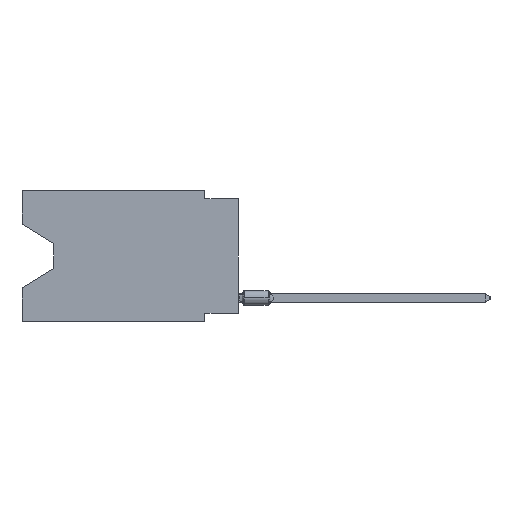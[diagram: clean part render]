
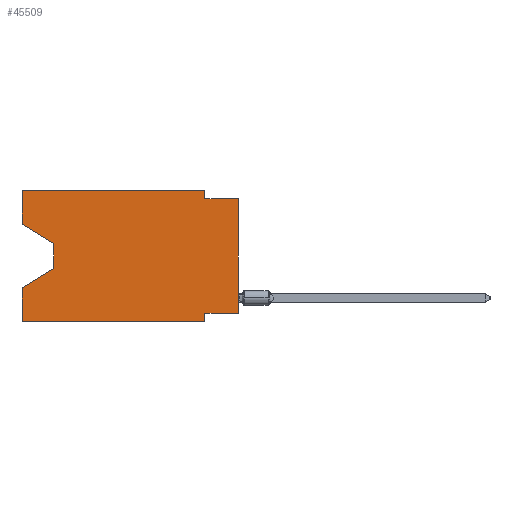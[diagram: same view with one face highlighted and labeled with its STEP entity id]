
A CAD part, left-side view. The second image highlights one B-rep face of the part: STEP entity #45509.
In plain terms, the highlighted planar face has unit normal (-1, 0, 0).
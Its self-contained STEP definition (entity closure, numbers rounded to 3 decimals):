
#133 = DIRECTION ( 'NONE',  ( 0., 0., -1. ) ) ;
#1844 = CARTESIAN_POINT ( 'NONE',  ( 0., 16.383, -2.546 ) ) ;
#2037 = ORIENTED_EDGE ( 'NONE', *, *, #19063, .T. ) ;
#2393 = CARTESIAN_POINT ( 'NONE',  ( 0., 0., -9.271 ) ) ;
#4251 = ORIENTED_EDGE ( 'NONE', *, *, #30617, .T. ) ;
#4697 = LINE ( 'NONE', #22172, #10840 ) ;
#5427 = VECTOR ( 'NONE', #28381, 1000. ) ;
#6247 = DIRECTION ( 'NONE',  ( 0., -1., 0. ) ) ;
#6946 = DIRECTION ( 'NONE',  ( 0., 1., 0. ) ) ;
#7631 = LINE ( 'NONE', #42583, #11906 ) ;
#7999 = CARTESIAN_POINT ( 'NONE',  ( 0., 16.383, 0. ) ) ;
#8309 = CARTESIAN_POINT ( 'NONE',  ( 0., 2.54, -9.906 ) ) ;
#9301 = LINE ( 'NONE', #1844, #46509 ) ;
#9688 = CARTESIAN_POINT ( 'NONE',  ( 0., 16.383, -2.546 ) ) ;
#10560 = LINE ( 'NONE', #45496, #26083 ) ;
#10840 = VECTOR ( 'NONE', #40492, 1000. ) ;
#11053 = ORIENTED_EDGE ( 'NONE', *, *, #41246, .F. ) ;
#11726 = DIRECTION ( 'NONE',  ( 0., 0., -1. ) ) ;
#11906 = VECTOR ( 'NONE', #54344, 1000. ) ;
#12915 = EDGE_CURVE ( 'NONE', #19166, #28089, #10560, .T. ) ;
#14670 = VECTOR ( 'NONE', #133, 1000. ) ;
#16348 = PLANE ( 'NONE',  #28451 ) ;
#17583 = VECTOR ( 'NONE', #33090, 1000. ) ;
#17687 = EDGE_CURVE ( 'NONE', #28089, #47008, #52532, .T. ) ;
#18298 = VERTEX_POINT ( 'NONE', #21334 ) ;
#19063 = EDGE_CURVE ( 'NONE', #41178, #54456, #50975, .T. ) ;
#19128 = CARTESIAN_POINT ( 'NONE',  ( 0., 2.54, 0. ) ) ;
#19166 = VERTEX_POINT ( 'NONE', #7999 ) ;
#19628 = LINE ( 'NONE', #37091, #17583 ) ;
#19798 = EDGE_CURVE ( 'NONE', #53933, #18298, #41623, .T. ) ;
#20090 = VECTOR ( 'NONE', #25200, 1000. ) ;
#20174 = VECTOR ( 'NONE', #6946, 1000. ) ;
#20194 = CARTESIAN_POINT ( 'NONE',  ( 0., 2.54, -0.635 ) ) ;
#20821 = CARTESIAN_POINT ( 'NONE',  ( 0., 16.383, -9.906 ) ) ;
#21334 = CARTESIAN_POINT ( 'NONE',  ( 0., 2.54, -9.271 ) ) ;
#21633 = VERTEX_POINT ( 'NONE', #9688 ) ;
#21896 = CARTESIAN_POINT ( 'NONE',  ( 0., 2.54, 0. ) ) ;
#22172 = CARTESIAN_POINT ( 'NONE',  ( 0., 0., -0.635 ) ) ;
#22261 = ORIENTED_EDGE ( 'NONE', *, *, #12915, .F. ) ;
#22433 = LINE ( 'NONE', #27019, #33358 ) ;
#22599 = CARTESIAN_POINT ( 'NONE',  ( 0., 16.383, -7.36 ) ) ;
#23037 = ORIENTED_EDGE ( 'NONE', *, *, #19798, .F. ) ;
#23476 = VERTEX_POINT ( 'NONE', #24173 ) ;
#23794 = LINE ( 'NONE', #28670, #5427 ) ;
#24173 = CARTESIAN_POINT ( 'NONE',  ( 0., 0., -0.635 ) ) ;
#24440 = EDGE_CURVE ( 'NONE', #53933, #23476, #23794, .T. ) ;
#24629 = CARTESIAN_POINT ( 'NONE',  ( 0., 16.383, 0. ) ) ;
#25200 = DIRECTION ( 'NONE',  ( 0., 0., 1. ) ) ;
#25782 = CARTESIAN_POINT ( 'NONE',  ( 0., 13.97, -5.893 ) ) ;
#26083 = VECTOR ( 'NONE', #6247, 1000. ) ;
#26792 = DIRECTION ( 'NONE',  ( 0., -0.855, -0.519 ) ) ;
#26874 = ORIENTED_EDGE ( 'NONE', *, *, #44849, .F. ) ;
#27019 = CARTESIAN_POINT ( 'NONE',  ( 0., 13.97, -4.013 ) ) ;
#27289 = EDGE_CURVE ( 'NONE', #18298, #51858, #42939, .T. ) ;
#27622 = CARTESIAN_POINT ( 'NONE',  ( 0., 13.97, -5.893 ) ) ;
#27803 = CARTESIAN_POINT ( 'NONE',  ( 0., 13.97, -4.013 ) ) ;
#27812 = ORIENTED_EDGE ( 'NONE', *, *, #27289, .F. ) ;
#28089 = VERTEX_POINT ( 'NONE', #19128 ) ;
#28381 = DIRECTION ( 'NONE',  ( 0., 0., 1. ) ) ;
#28451 = AXIS2_PLACEMENT_3D ( 'NONE', #33826, #45873, #51299 ) ;
#28670 = CARTESIAN_POINT ( 'NONE',  ( 0., 0., 0. ) ) ;
#30617 = EDGE_CURVE ( 'NONE', #43696, #51858, #19628, .T. ) ;
#33090 = DIRECTION ( 'NONE',  ( 0., -1., 0. ) ) ;
#33358 = VECTOR ( 'NONE', #40167, 1000. ) ;
#33826 = CARTESIAN_POINT ( 'NONE',  ( 0., 16.383, 0. ) ) ;
#34438 = EDGE_CURVE ( 'NONE', #46188, #41178, #22433, .T. ) ;
#37091 = CARTESIAN_POINT ( 'NONE',  ( 0., 16.383, -9.906 ) ) ;
#37950 = ORIENTED_EDGE ( 'NONE', *, *, #38892, .T. ) ;
#38069 = LINE ( 'NONE', #24629, #20090 ) ;
#38892 = EDGE_CURVE ( 'NONE', #21633, #46188, #9301, .T. ) ;
#39300 = ORIENTED_EDGE ( 'NONE', *, *, #24440, .T. ) ;
#39445 = VECTOR ( 'NONE', #47525, 1000. ) ;
#40167 = DIRECTION ( 'NONE',  ( 0., 0., -1. ) ) ;
#40410 = ORIENTED_EDGE ( 'NONE', *, *, #34438, .T. ) ;
#40492 = DIRECTION ( 'NONE',  ( 0., -1., 0. ) ) ;
#41178 = VERTEX_POINT ( 'NONE', #27622 ) ;
#41246 = EDGE_CURVE ( 'NONE', #47008, #23476, #4697, .T. ) ;
#41623 = LINE ( 'NONE', #2393, #20174 ) ;
#42583 = CARTESIAN_POINT ( 'NONE',  ( 0., 16.383, 0. ) ) ;
#42939 = LINE ( 'NONE', #50960, #55738 ) ;
#43696 = VERTEX_POINT ( 'NONE', #20821 ) ;
#44411 = EDGE_CURVE ( 'NONE', #43696, #54456, #38069, .T. ) ;
#44849 = EDGE_CURVE ( 'NONE', #21633, #19166, #7631, .T. ) ;
#45496 = CARTESIAN_POINT ( 'NONE',  ( 0., 16.383, 0. ) ) ;
#45509 = ADVANCED_FACE ( 'NONE', ( #55577 ), #16348, .F. ) ;
#45873 = DIRECTION ( 'NONE',  ( 1., 0., 0. ) ) ;
#46188 = VERTEX_POINT ( 'NONE', #27803 ) ;
#46509 = VECTOR ( 'NONE', #26792, 1000. ) ;
#47008 = VERTEX_POINT ( 'NONE', #20194 ) ;
#47171 = ORIENTED_EDGE ( 'NONE', *, *, #44411, .F. ) ;
#47525 = DIRECTION ( 'NONE',  ( 0., 0.855, -0.519 ) ) ;
#50960 = CARTESIAN_POINT ( 'NONE',  ( 0., 2.54, -9.906 ) ) ;
#50975 = LINE ( 'NONE', #25782, #39445 ) ;
#51299 = DIRECTION ( 'NONE',  ( 0., 0., -1. ) ) ;
#51858 = VERTEX_POINT ( 'NONE', #8309 ) ;
#52163 = CARTESIAN_POINT ( 'NONE',  ( 0., 0., -9.271 ) ) ;
#52532 = LINE ( 'NONE', #21896, #14670 ) ;
#53933 = VERTEX_POINT ( 'NONE', #52163 ) ;
#54092 = ORIENTED_EDGE ( 'NONE', *, *, #17687, .F. ) ;
#54243 = EDGE_LOOP ( 'NONE', ( #37950, #40410, #2037, #47171, #4251, #27812, #23037, #39300, #11053, #54092, #22261, #26874 ) ) ;
#54344 = DIRECTION ( 'NONE',  ( 0., 0., 1. ) ) ;
#54456 = VERTEX_POINT ( 'NONE', #22599 ) ;
#55577 = FACE_OUTER_BOUND ( 'NONE', #54243, .T. ) ;
#55738 = VECTOR ( 'NONE', #11726, 1000. ) ;
